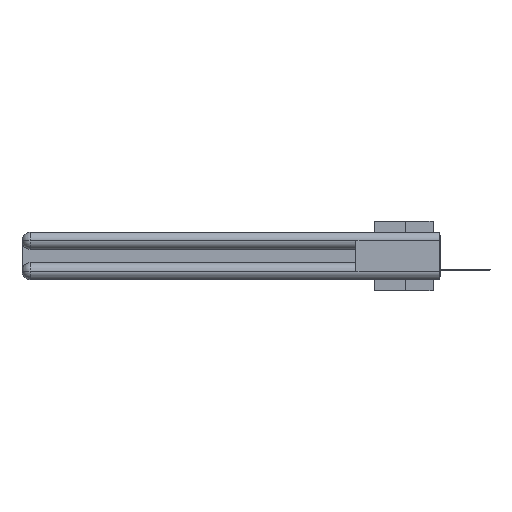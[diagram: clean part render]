
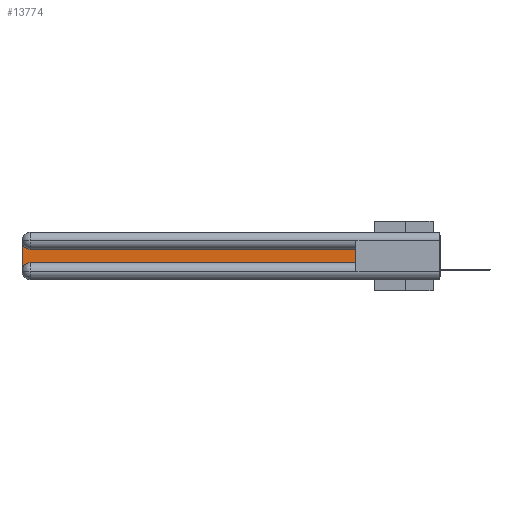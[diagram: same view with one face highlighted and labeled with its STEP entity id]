
A CAD part, left-side view. The second image highlights one B-rep face of the part: STEP entity #13774.
In plain terms, the highlighted planar face has unit normal (-1, 0, 0).
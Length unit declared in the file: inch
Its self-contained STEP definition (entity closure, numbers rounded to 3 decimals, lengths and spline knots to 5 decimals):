
#190 = CARTESIAN_POINT ( 'NONE',  ( 0.075, 0.6, -0.1225 ) ) ;
#539 = DIRECTION ( 'NONE',  ( 1., 0., 0. ) ) ;
#544 = CARTESIAN_POINT ( 'NONE',  ( 0.075, 3., -0.1225 ) ) ;
#747 = PLANE ( 'NONE',  #21483 ) ;
#1197 = AXIS2_PLACEMENT_3D ( 'NONE', #29283, #539, #28331 ) ;
#1446 = CARTESIAN_POINT ( 'NONE',  ( 0.075, 3., -0.2175 ) ) ;
#2132 = VECTOR ( 'NONE', #38363, 39.37008 ) ;
#3791 = FACE_OUTER_BOUND ( 'NONE', #35142, .T. ) ;
#5260 = LINE ( 'NONE', #29989, #28651 ) ;
#6839 = ORIENTED_EDGE ( 'NONE', *, *, #8849, .T. ) ;
#7163 = VERTEX_POINT ( 'NONE', #14788 ) ;
#7325 = CARTESIAN_POINT ( 'NONE',  ( 0.075, 2.94, -0.0625 ) ) ;
#7338 = LINE ( 'NONE', #1446, #11444 ) ;
#7911 = DIRECTION ( 'NONE',  ( 0., 0., 1. ) ) ;
#8849 = EDGE_CURVE ( 'NONE', #7163, #17510, #7338, .T. ) ;
#10981 = EDGE_CURVE ( 'NONE', #17510, #35604, #17374, .T. ) ;
#11444 = VECTOR ( 'NONE', #13810, 39.37008 ) ;
#11693 = VERTEX_POINT ( 'NONE', #13210 ) ;
#11995 = EDGE_CURVE ( 'NONE', #19543, #31160, #27985, .T. ) ;
#12572 = DIRECTION ( 'NONE',  ( 0., 1., 0. ) ) ;
#13210 = CARTESIAN_POINT ( 'NONE',  ( 0.075, 0.6, -0.2175 ) ) ;
#13774 = ADVANCED_FACE ( 'NONE', ( #3791 ), #747, .F. ) ;
#13810 = DIRECTION ( 'NONE',  ( 0., 0., -1. ) ) ;
#14788 = CARTESIAN_POINT ( 'NONE',  ( 0.075, 3., -0.0625 ) ) ;
#15066 = LINE ( 'NONE', #22361, #2132 ) ;
#15347 = ORIENTED_EDGE ( 'NONE', *, *, #11995, .T. ) ;
#17374 = CIRCLE ( 'NONE', #1197, 0.06 ) ;
#17510 = VERTEX_POINT ( 'NONE', #39864 ) ;
#19009 = DIRECTION ( 'NONE',  ( 0., 0., -1. ) ) ;
#19543 = VERTEX_POINT ( 'NONE', #25871 ) ;
#19668 = DIRECTION ( 'NONE',  ( 0., 0., -1. ) ) ;
#21483 = AXIS2_PLACEMENT_3D ( 'NONE', #544, #22050, #19009 ) ;
#22050 = DIRECTION ( 'NONE',  ( 1., 0., 0. ) ) ;
#22361 = CARTESIAN_POINT ( 'NONE',  ( 0.075, 0.6, -0.2175 ) ) ;
#23807 = ORIENTED_EDGE ( 'NONE', *, *, #24409, .T. ) ;
#24409 = EDGE_CURVE ( 'NONE', #11693, #19543, #5260, .T. ) ;
#24561 = ORIENTED_EDGE ( 'NONE', *, *, #10981, .T. ) ;
#24871 = CARTESIAN_POINT ( 'NONE',  ( 0.075, 2.94, -0.2175 ) ) ;
#25057 = EDGE_CURVE ( 'NONE', #35604, #11693, #15066, .T. ) ;
#25871 = CARTESIAN_POINT ( 'NONE',  ( 0.075, 0.6, -0.1225 ) ) ;
#26889 = EDGE_CURVE ( 'NONE', #31160, #7163, #27803, .T. ) ;
#27390 = CARTESIAN_POINT ( 'NONE',  ( 0.075, 2.94, -0.1225 ) ) ;
#27803 = CIRCLE ( 'NONE', #38156, 0.06 ) ;
#27985 = LINE ( 'NONE', #190, #34302 ) ;
#28331 = DIRECTION ( 'NONE',  ( 0., 0., -1. ) ) ;
#28406 = ORIENTED_EDGE ( 'NONE', *, *, #25057, .T. ) ;
#28611 = DIRECTION ( 'NONE',  ( 1., 0., 0. ) ) ;
#28651 = VECTOR ( 'NONE', #7911, 39.37008 ) ;
#29283 = CARTESIAN_POINT ( 'NONE',  ( 0.075, 2.94, -0.2775 ) ) ;
#29989 = CARTESIAN_POINT ( 'NONE',  ( 0.075, 0.6, -0.2175 ) ) ;
#31160 = VERTEX_POINT ( 'NONE', #27390 ) ;
#32796 = ORIENTED_EDGE ( 'NONE', *, *, #26889, .T. ) ;
#34302 = VECTOR ( 'NONE', #12572, 39.37008 ) ;
#35142 = EDGE_LOOP ( 'NONE', ( #15347, #32796, #6839, #24561, #28406, #23807 ) ) ;
#35604 = VERTEX_POINT ( 'NONE', #24871 ) ;
#38156 = AXIS2_PLACEMENT_3D ( 'NONE', #7325, #28611, #19668 ) ;
#38363 = DIRECTION ( 'NONE',  ( 0., -1., 0. ) ) ;
#39864 = CARTESIAN_POINT ( 'NONE',  ( 0.075, 3., -0.2775 ) ) ;
